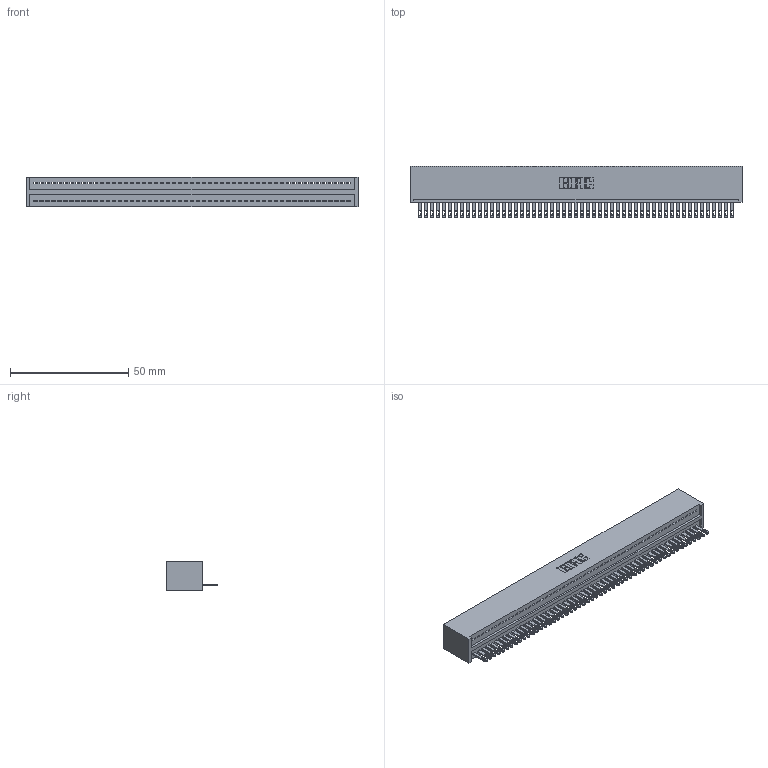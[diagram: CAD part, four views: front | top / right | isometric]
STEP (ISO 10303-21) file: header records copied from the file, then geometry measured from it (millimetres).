
FILE_DESCRIPTION (( 'STEP AP203' ), '1' );
FILE_NAME ('325-053-500-101.STEP', '2020-02-25T00:35:13', ( '' ), ( '' ), 'SwSTEP 2.0', 'SolidWorks 2016', '' );
FILE_SCHEMA (( 'CONFIG_CONTROL_DESIGN' ));
Length unit declared in the file: inch
Products named in the file (3): 325-292-001_325-293-100; 325 Part_Lugless; 325-053-500-101
Assembly tree (54 placements, depth 2):
  325-053-500-101
    325 Part_Lugless
    325-292-001_325-293-100  x53
Bounding box: 140.26 x 21.84 x 12.45 mm (x, y, z)
Volume: 18497 mm3; surface area: 21009 mm2
Topology: 54 solids, 54 shells, 2968 faces, 9191 edges, 6126 vertices
Faces by surface type: plane 1974, cylinder 994
Entity records: 30631 total; most frequent: CARTESIAN_POINT 5289, ORIENTED_EDGE 5278, DIRECTION 4433, EDGE_CURVE 2639, VECTOR 2515, LINE 2515, VERTEX_POINT 1758, AXIS2_PLACEMENT_3D 959
